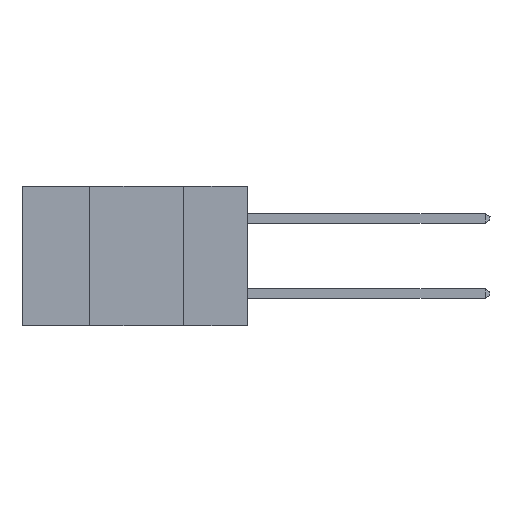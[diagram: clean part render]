
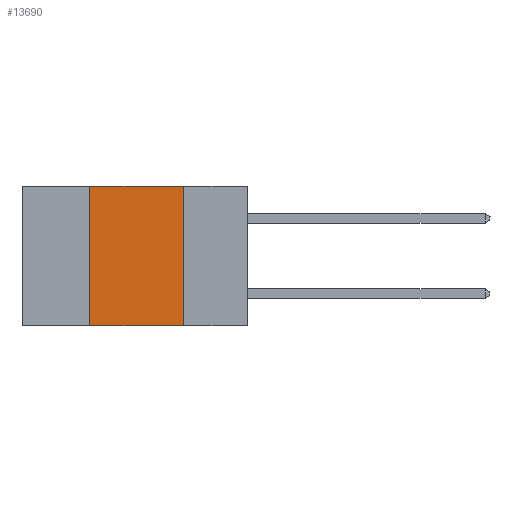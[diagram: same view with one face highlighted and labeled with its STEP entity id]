
A CAD part, left-side view. The second image highlights one B-rep face of the part: STEP entity #13690.
In plain terms, the highlighted planar face has unit normal (-1, 0, 0).
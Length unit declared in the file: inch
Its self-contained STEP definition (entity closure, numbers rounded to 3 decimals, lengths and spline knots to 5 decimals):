
#162 = EDGE_CURVE ( 'NONE', #269, #7522, #3804, .T. ) ;
#269 = VERTEX_POINT ( 'NONE', #7356 ) ;
#387 = DIRECTION ( 'NONE',  ( 0., 0., -1. ) ) ;
#861 = ORIENTED_EDGE ( 'NONE', *, *, #16151, .F. ) ;
#1981 = DIRECTION ( 'NONE',  ( 0., -1., 0. ) ) ;
#2131 = LINE ( 'NONE', #13303, #12047 ) ;
#2424 = LINE ( 'NONE', #14417, #19237 ) ;
#2559 = VECTOR ( 'NONE', #1981, 39.37008 ) ;
#2903 = VERTEX_POINT ( 'NONE', #10830 ) ;
#3620 = EDGE_LOOP ( 'NONE', ( #861, #5810, #20924, #13254 ) ) ;
#3804 = LINE ( 'NONE', #18177, #2559 ) ;
#3993 = PLANE ( 'NONE',  #20480 ) ;
#4062 = DIRECTION ( 'NONE',  ( 0., 0., -1. ) ) ;
#4533 = CARTESIAN_POINT ( 'NONE',  ( 0., 0.6, -0.37 ) ) ;
#4603 = DIRECTION ( 'NONE',  ( 0., -1., 0. ) ) ;
#5810 = ORIENTED_EDGE ( 'NONE', *, *, #162, .F. ) ;
#7356 = CARTESIAN_POINT ( 'NONE',  ( 0., 0.42, 0. ) ) ;
#7522 = VERTEX_POINT ( 'NONE', #20059 ) ;
#7931 = LINE ( 'NONE', #4533, #8202 ) ;
#8202 = VECTOR ( 'NONE', #4603, 39.37008 ) ;
#10830 = CARTESIAN_POINT ( 'NONE',  ( 0., 0.42, -0.37 ) ) ;
#11369 = FACE_OUTER_BOUND ( 'NONE', #3620, .T. ) ;
#12047 = VECTOR ( 'NONE', #387, 39.37008 ) ;
#12659 = CARTESIAN_POINT ( 'NONE',  ( 0., 0.17, -0.37 ) ) ;
#13254 = ORIENTED_EDGE ( 'NONE', *, *, #19757, .T. ) ;
#13303 = CARTESIAN_POINT ( 'NONE',  ( 0., 0.17, 0. ) ) ;
#13690 = ADVANCED_FACE ( 'NONE', ( #11369 ), #3993, .F. ) ;
#14417 = CARTESIAN_POINT ( 'NONE',  ( 0., 0.42, 0. ) ) ;
#14562 = DIRECTION ( 'NONE',  ( 0., 0., 1. ) ) ;
#16151 = EDGE_CURVE ( 'NONE', #7522, #20725, #2131, .T. ) ;
#16934 = DIRECTION ( 'NONE',  ( 1., 0., 0. ) ) ;
#18177 = CARTESIAN_POINT ( 'NONE',  ( 0., 0.6, 0. ) ) ;
#18640 = CARTESIAN_POINT ( 'NONE',  ( 0., 0.6, 0. ) ) ;
#18860 = EDGE_CURVE ( 'NONE', #2903, #269, #2424, .T. ) ;
#19237 = VECTOR ( 'NONE', #14562, 39.37008 ) ;
#19757 = EDGE_CURVE ( 'NONE', #2903, #20725, #7931, .T. ) ;
#20059 = CARTESIAN_POINT ( 'NONE',  ( 0., 0.17, 0. ) ) ;
#20480 = AXIS2_PLACEMENT_3D ( 'NONE', #18640, #16934, #4062 ) ;
#20725 = VERTEX_POINT ( 'NONE', #12659 ) ;
#20924 = ORIENTED_EDGE ( 'NONE', *, *, #18860, .F. ) ;
